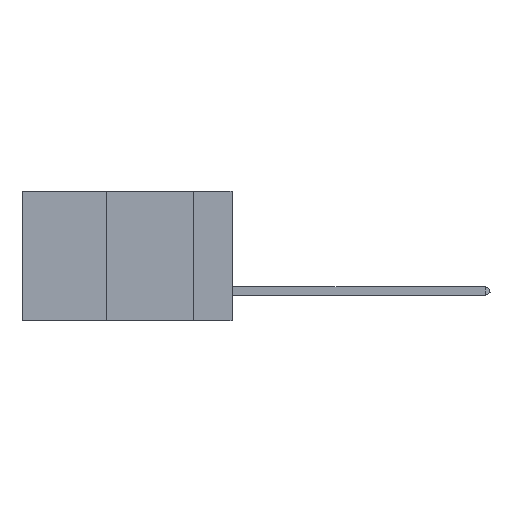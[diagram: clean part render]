
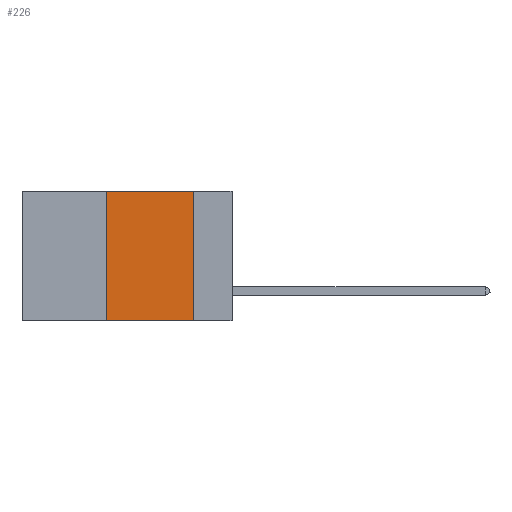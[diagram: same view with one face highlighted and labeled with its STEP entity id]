
A CAD part, left-side view. The second image highlights one B-rep face of the part: STEP entity #226.
In plain terms, the highlighted planar face has unit normal (-1, 0, 0).
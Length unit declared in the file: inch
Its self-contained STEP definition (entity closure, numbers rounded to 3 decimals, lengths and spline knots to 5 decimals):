
#141 = FACE_OUTER_BOUND ( 'NONE', #11397, .T. ) ;
#226 = ADVANCED_FACE ( 'NONE', ( #141 ), #10638, .F. ) ;
#661 = VERTEX_POINT ( 'NONE', #12699 ) ;
#684 = CARTESIAN_POINT ( 'NONE',  ( 0., 0.6, 0. ) ) ;
#1068 = DIRECTION ( 'NONE',  ( 0., -1., 0. ) ) ;
#2782 = VECTOR ( 'NONE', #10698, 39.37008 ) ;
#2802 = CARTESIAN_POINT ( 'NONE',  ( 0., 0.6, 0. ) ) ;
#3006 = DIRECTION ( 'NONE',  ( 0., 0., -1. ) ) ;
#3107 = VECTOR ( 'NONE', #1068, 39.37008 ) ;
#3790 = VERTEX_POINT ( 'NONE', #12691 ) ;
#4047 = DIRECTION ( 'NONE',  ( 0., 0., -1. ) ) ;
#4461 = ORIENTED_EDGE ( 'NONE', *, *, #14215, .F. ) ;
#5194 = EDGE_CURVE ( 'NONE', #3790, #8825, #12378, .T. ) ;
#5235 = CARTESIAN_POINT ( 'NONE',  ( 0., 0.36, 0. ) ) ;
#5567 = VECTOR ( 'NONE', #14082, 39.37008 ) ;
#6060 = ORIENTED_EDGE ( 'NONE', *, *, #10093, .F. ) ;
#6284 = CARTESIAN_POINT ( 'NONE',  ( 0., 0.11, 0. ) ) ;
#6521 = CARTESIAN_POINT ( 'NONE',  ( 0., 0.6, -0.37 ) ) ;
#8609 = LINE ( 'NONE', #6521, #3107 ) ;
#8825 = VERTEX_POINT ( 'NONE', #12019 ) ;
#9262 = AXIS2_PLACEMENT_3D ( 'NONE', #2802, #13816, #4047 ) ;
#9442 = CARTESIAN_POINT ( 'NONE',  ( 0., 0.36, -0.37 ) ) ;
#10093 = EDGE_CURVE ( 'NONE', #11363, #661, #10184, .T. ) ;
#10184 = LINE ( 'NONE', #5235, #5567 ) ;
#10638 = PLANE ( 'NONE',  #9262 ) ;
#10698 = DIRECTION ( 'NONE',  ( 0., -1., 0. ) ) ;
#10839 = EDGE_CURVE ( 'NONE', #11363, #8825, #8609, .T. ) ;
#11363 = VERTEX_POINT ( 'NONE', #9442 ) ;
#11397 = EDGE_LOOP ( 'NONE', ( #12388, #4461, #6060, #12668 ) ) ;
#12019 = CARTESIAN_POINT ( 'NONE',  ( 0., 0.11, -0.37 ) ) ;
#12378 = LINE ( 'NONE', #6284, #14137 ) ;
#12388 = ORIENTED_EDGE ( 'NONE', *, *, #5194, .F. ) ;
#12668 = ORIENTED_EDGE ( 'NONE', *, *, #10839, .T. ) ;
#12691 = CARTESIAN_POINT ( 'NONE',  ( 0., 0.11, 0. ) ) ;
#12699 = CARTESIAN_POINT ( 'NONE',  ( 0., 0.36, 0. ) ) ;
#13816 = DIRECTION ( 'NONE',  ( 1., 0., 0. ) ) ;
#13854 = LINE ( 'NONE', #684, #2782 ) ;
#14082 = DIRECTION ( 'NONE',  ( 0., 0., 1. ) ) ;
#14137 = VECTOR ( 'NONE', #3006, 39.37008 ) ;
#14215 = EDGE_CURVE ( 'NONE', #661, #3790, #13854, .T. ) ;
